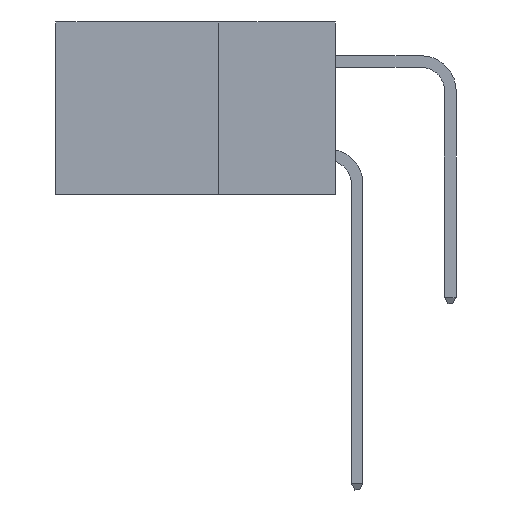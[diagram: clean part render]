
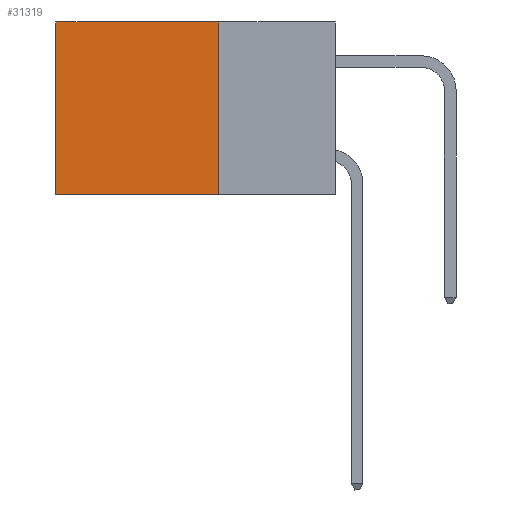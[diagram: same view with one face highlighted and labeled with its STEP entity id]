
A CAD part, left-side view. The second image highlights one B-rep face of the part: STEP entity #31319.
In plain terms, the highlighted planar face has unit normal (-1, 0, 0).
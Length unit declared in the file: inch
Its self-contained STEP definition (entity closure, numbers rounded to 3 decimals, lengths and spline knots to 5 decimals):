
#508 = CARTESIAN_POINT ( 'NONE',  ( 0.2875, 0.25, 0. ) ) ;
#2975 = DIRECTION ( 'NONE',  ( 0., 0., -1. ) ) ;
#3928 = DIRECTION ( 'NONE',  ( 0., 0., -1. ) ) ;
#4334 = LINE ( 'NONE', #9015, #25938 ) ;
#4703 = EDGE_LOOP ( 'NONE', ( #39923, #31560, #9585, #7480 ) ) ;
#5559 = AXIS2_PLACEMENT_3D ( 'NONE', #6269, #9594, #2975 ) ;
#6269 = CARTESIAN_POINT ( 'NONE',  ( 0.2875, 0.25, 0. ) ) ;
#6542 = FACE_OUTER_BOUND ( 'NONE', #4703, .T. ) ;
#7204 = LINE ( 'NONE', #508, #39928 ) ;
#7267 = VERTEX_POINT ( 'NONE', #37464 ) ;
#7422 = CARTESIAN_POINT ( 'NONE',  ( 0.2875, 0.25, -0.37 ) ) ;
#7480 = ORIENTED_EDGE ( 'NONE', *, *, #39867, .T. ) ;
#7581 = LINE ( 'NONE', #15096, #25738 ) ;
#9015 = CARTESIAN_POINT ( 'NONE',  ( 0.2875, 0.6, 0. ) ) ;
#9557 = DIRECTION ( 'NONE',  ( 0., 0., -1. ) ) ;
#9585 = ORIENTED_EDGE ( 'NONE', *, *, #28722, .F. ) ;
#9594 = DIRECTION ( 'NONE',  ( 1., 0., 0. ) ) ;
#9865 = VERTEX_POINT ( 'NONE', #28902 ) ;
#15096 = CARTESIAN_POINT ( 'NONE',  ( 0.2875, 0.25, 0. ) ) ;
#20945 = DIRECTION ( 'NONE',  ( 0., 1., 0. ) ) ;
#23906 = CARTESIAN_POINT ( 'NONE',  ( 0.2875, 0.6, -0.37 ) ) ;
#25041 = EDGE_CURVE ( 'NONE', #9865, #38582, #28499, .T. ) ;
#25185 = PLANE ( 'NONE',  #5559 ) ;
#25738 = VECTOR ( 'NONE', #20945, 39.37008 ) ;
#25938 = VECTOR ( 'NONE', #9557, 39.37008 ) ;
#26087 = EDGE_CURVE ( 'NONE', #26666, #38582, #4334, .T. ) ;
#26666 = VERTEX_POINT ( 'NONE', #31450 ) ;
#27516 = VECTOR ( 'NONE', #29718, 39.37008 ) ;
#28499 = LINE ( 'NONE', #7422, #27516 ) ;
#28722 = EDGE_CURVE ( 'NONE', #7267, #9865, #7204, .T. ) ;
#28902 = CARTESIAN_POINT ( 'NONE',  ( 0.2875, 0.25, -0.37 ) ) ;
#29718 = DIRECTION ( 'NONE',  ( 0., 1., 0. ) ) ;
#31319 = ADVANCED_FACE ( 'NONE', ( #6542 ), #25185, .F. ) ;
#31450 = CARTESIAN_POINT ( 'NONE',  ( 0.2875, 0.6, 0. ) ) ;
#31560 = ORIENTED_EDGE ( 'NONE', *, *, #25041, .F. ) ;
#37464 = CARTESIAN_POINT ( 'NONE',  ( 0.2875, 0.25, 0. ) ) ;
#38582 = VERTEX_POINT ( 'NONE', #23906 ) ;
#39867 = EDGE_CURVE ( 'NONE', #7267, #26666, #7581, .T. ) ;
#39923 = ORIENTED_EDGE ( 'NONE', *, *, #26087, .T. ) ;
#39928 = VECTOR ( 'NONE', #3928, 39.37008 ) ;
